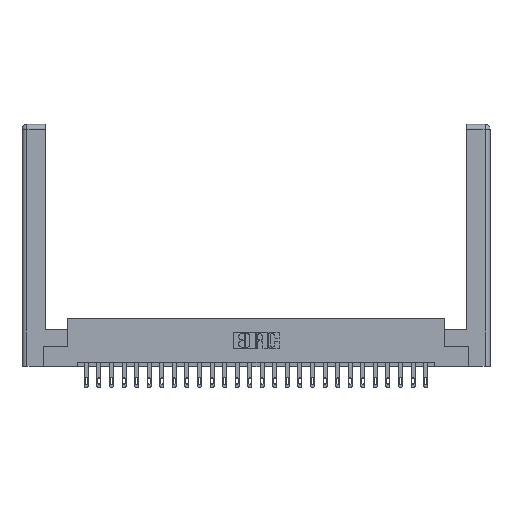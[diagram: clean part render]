
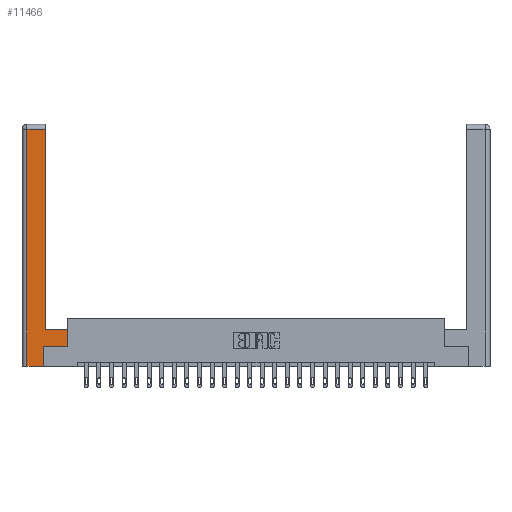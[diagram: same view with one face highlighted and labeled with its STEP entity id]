
A CAD part, top view. The second image highlights one B-rep face of the part: STEP entity #11466.
In plain terms, the highlighted planar face has unit normal (0, 0, 1).
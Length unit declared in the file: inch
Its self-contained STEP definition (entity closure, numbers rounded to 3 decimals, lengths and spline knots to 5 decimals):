
#200 = VERTEX_POINT ( 'NONE', #15398 ) ;
#274 = CARTESIAN_POINT ( 'NONE',  ( 0.0615, 2.94, 0. ) ) ;
#421 = LINE ( 'NONE', #17517, #3861 ) ;
#460 = CARTESIAN_POINT ( 'NONE',  ( 0.295, 0.45, 0. ) ) ;
#567 = EDGE_CURVE ( 'NONE', #14604, #14135, #6905, .T. ) ;
#765 = PLANE ( 'NONE',  #19508 ) ;
#1002 = VERTEX_POINT ( 'NONE', #24241 ) ;
#1172 = EDGE_CURVE ( 'NONE', #14135, #1002, #5304, .T. ) ;
#1583 = VERTEX_POINT ( 'NONE', #15415 ) ;
#2127 = CARTESIAN_POINT ( 'NONE',  ( 0.265, 0., 0. ) ) ;
#2350 = DIRECTION ( 'NONE',  ( 0., 0., -1. ) ) ;
#2564 = DIRECTION ( 'NONE',  ( -1., 0., 0. ) ) ;
#3003 = CARTESIAN_POINT ( 'NONE',  ( 0.0615, 0., 0. ) ) ;
#3497 = VECTOR ( 'NONE', #14357, 39.37008 ) ;
#3861 = VECTOR ( 'NONE', #21632, 39.37008 ) ;
#4393 = FACE_OUTER_BOUND ( 'NONE', #23648, .T. ) ;
#4421 = CARTESIAN_POINT ( 'NONE',  ( 0.265, 0., 0. ) ) ;
#4903 = VECTOR ( 'NONE', #11117, 39.37008 ) ;
#5304 = LINE ( 'NONE', #460, #15399 ) ;
#5579 = ORIENTED_EDGE ( 'NONE', *, *, #9815, .T. ) ;
#5636 = VECTOR ( 'NONE', #18811, 39.37008 ) ;
#6242 = CARTESIAN_POINT ( 'NONE',  ( 0.295, 3., 0. ) ) ;
#6585 = VERTEX_POINT ( 'NONE', #17210 ) ;
#6905 = LINE ( 'NONE', #20827, #5636 ) ;
#6932 = LINE ( 'NONE', #6242, #19215 ) ;
#7195 = EDGE_CURVE ( 'NONE', #1583, #6585, #25089, .T. ) ;
#8412 = CARTESIAN_POINT ( 'NONE',  ( 0.565, 0.245, 0. ) ) ;
#8781 = VECTOR ( 'NONE', #10515, 39.37008 ) ;
#9467 = ORIENTED_EDGE ( 'NONE', *, *, #1172, .T. ) ;
#9815 = EDGE_CURVE ( 'NONE', #24965, #14604, #421, .T. ) ;
#10515 = DIRECTION ( 'NONE',  ( 1., 0., 0. ) ) ;
#10825 = DIRECTION ( 'NONE',  ( 0., 1., 0. ) ) ;
#11117 = DIRECTION ( 'NONE',  ( 0., -1., 0. ) ) ;
#11372 = EDGE_CURVE ( 'NONE', #1002, #200, #6932, .T. ) ;
#11466 = ADVANCED_FACE ( 'NONE', ( #4393 ), #765, .F. ) ;
#13243 = ORIENTED_EDGE ( 'NONE', *, *, #7195, .T. ) ;
#14135 = VERTEX_POINT ( 'NONE', #15388 ) ;
#14357 = DIRECTION ( 'NONE',  ( -1., 0., 0. ) ) ;
#14604 = VERTEX_POINT ( 'NONE', #8412 ) ;
#15388 = CARTESIAN_POINT ( 'NONE',  ( 0.565, 0.45, 0. ) ) ;
#15398 = CARTESIAN_POINT ( 'NONE',  ( 0.295, 2.94, 0. ) ) ;
#15399 = VECTOR ( 'NONE', #2564, 39.37008 ) ;
#15415 = CARTESIAN_POINT ( 'NONE',  ( 0.0615, 2.94, 0. ) ) ;
#15906 = ORIENTED_EDGE ( 'NONE', *, *, #19016, .T. ) ;
#16624 = EDGE_CURVE ( 'NONE', #6585, #19993, #21996, .T. ) ;
#17210 = CARTESIAN_POINT ( 'NONE',  ( 0.0615, 0., 0. ) ) ;
#17517 = CARTESIAN_POINT ( 'NONE',  ( 0.565, 0.245, 0. ) ) ;
#18333 = LINE ( 'NONE', #274, #3497 ) ;
#18651 = DIRECTION ( 'NONE',  ( -1., 0., 0. ) ) ;
#18739 = VECTOR ( 'NONE', #10825, 39.37008 ) ;
#18811 = DIRECTION ( 'NONE',  ( 0., 1., 0. ) ) ;
#19016 = EDGE_CURVE ( 'NONE', #19993, #24965, #19372, .T. ) ;
#19215 = VECTOR ( 'NONE', #20584, 39.37008 ) ;
#19372 = LINE ( 'NONE', #22899, #18739 ) ;
#19508 = AXIS2_PLACEMENT_3D ( 'NONE', #22615, #2350, #18651 ) ;
#19993 = VERTEX_POINT ( 'NONE', #2127 ) ;
#20584 = DIRECTION ( 'NONE',  ( 0., 1., 0. ) ) ;
#20827 = CARTESIAN_POINT ( 'NONE',  ( 0.565, 0.45, 0. ) ) ;
#21205 = ORIENTED_EDGE ( 'NONE', *, *, #21473, .T. ) ;
#21341 = ORIENTED_EDGE ( 'NONE', *, *, #567, .T. ) ;
#21473 = EDGE_CURVE ( 'NONE', #200, #1583, #18333, .T. ) ;
#21632 = DIRECTION ( 'NONE',  ( 1., 0., 0. ) ) ;
#21996 = LINE ( 'NONE', #4421, #8781 ) ;
#22615 = CARTESIAN_POINT ( 'NONE',  ( 0., 0., 0. ) ) ;
#22620 = CARTESIAN_POINT ( 'NONE',  ( 0.265, 0.245, 0. ) ) ;
#22899 = CARTESIAN_POINT ( 'NONE',  ( 0.265, 0.245, 0. ) ) ;
#23648 = EDGE_LOOP ( 'NONE', ( #25406, #21205, #13243, #25601, #15906, #5579, #21341, #9467 ) ) ;
#24241 = CARTESIAN_POINT ( 'NONE',  ( 0.295, 0.45, 0. ) ) ;
#24965 = VERTEX_POINT ( 'NONE', #22620 ) ;
#25089 = LINE ( 'NONE', #3003, #4903 ) ;
#25406 = ORIENTED_EDGE ( 'NONE', *, *, #11372, .T. ) ;
#25601 = ORIENTED_EDGE ( 'NONE', *, *, #16624, .T. ) ;
